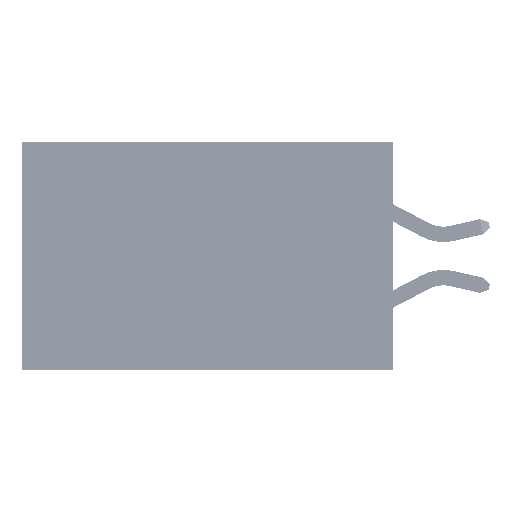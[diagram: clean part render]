
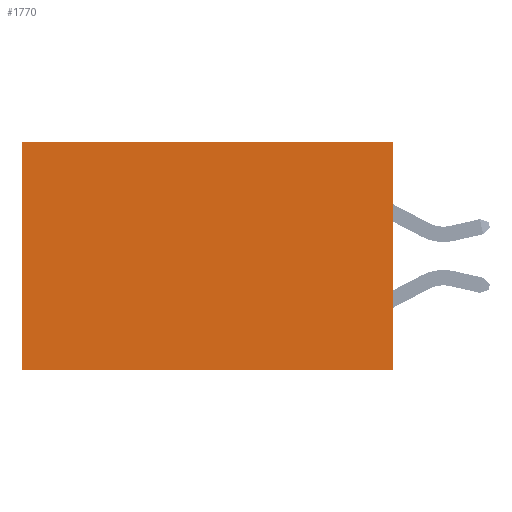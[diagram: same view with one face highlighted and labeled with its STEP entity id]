
A CAD part, left-side view. The second image highlights one B-rep face of the part: STEP entity #1770.
In plain terms, the highlighted planar face has unit normal (-1, 0, 0).
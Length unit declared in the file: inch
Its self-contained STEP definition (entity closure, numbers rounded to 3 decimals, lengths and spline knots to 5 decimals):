
#869 = VECTOR ( 'NONE', #29882, 39.37008 ) ;
#1770 = ADVANCED_FACE ( 'NONE', ( #36019 ), #12127, .F. ) ;
#2548 = EDGE_CURVE ( 'NONE', #43400, #11097, #41888, .T. ) ;
#6231 = CARTESIAN_POINT ( 'NONE',  ( 0.2875, 0.6, 0. ) ) ;
#7928 = EDGE_CURVE ( 'NONE', #30086, #43400, #29965, .T. ) ;
#8043 = EDGE_CURVE ( 'NONE', #30086, #38669, #17926, .T. ) ;
#9518 = VECTOR ( 'NONE', #36520, 39.37008 ) ;
#11097 = VERTEX_POINT ( 'NONE', #26124 ) ;
#11501 = EDGE_LOOP ( 'NONE', ( #35897, #20294, #34209, #25399 ) ) ;
#12127 = PLANE ( 'NONE',  #30588 ) ;
#17926 = LINE ( 'NONE', #28607, #9518 ) ;
#19720 = DIRECTION ( 'NONE',  ( 1., 0., 0. ) ) ;
#20294 = ORIENTED_EDGE ( 'NONE', *, *, #21108, .F. ) ;
#21108 = EDGE_CURVE ( 'NONE', #38669, #11097, #23764, .T. ) ;
#23764 = LINE ( 'NONE', #44851, #869 ) ;
#24514 = CARTESIAN_POINT ( 'NONE',  ( 0.2875, 0., -0.37 ) ) ;
#25399 = ORIENTED_EDGE ( 'NONE', *, *, #7928, .T. ) ;
#26124 = CARTESIAN_POINT ( 'NONE',  ( 0.2875, 0.6, -0.37 ) ) ;
#26771 = DIRECTION ( 'NONE',  ( 0., 0., -1. ) ) ;
#27889 = CARTESIAN_POINT ( 'NONE',  ( 0.2875, 0., 0. ) ) ;
#28607 = CARTESIAN_POINT ( 'NONE',  ( 0.2875, 0., 0. ) ) ;
#29882 = DIRECTION ( 'NONE',  ( 0., 1., 0. ) ) ;
#29965 = LINE ( 'NONE', #46790, #38418 ) ;
#30086 = VERTEX_POINT ( 'NONE', #27889 ) ;
#30588 = AXIS2_PLACEMENT_3D ( 'NONE', #46478, #19720, #26771 ) ;
#31828 = DIRECTION ( 'NONE',  ( 0., 1., 0. ) ) ;
#34209 = ORIENTED_EDGE ( 'NONE', *, *, #8043, .F. ) ;
#35166 = CARTESIAN_POINT ( 'NONE',  ( 0.2875, 0.6, 0. ) ) ;
#35897 = ORIENTED_EDGE ( 'NONE', *, *, #2548, .T. ) ;
#36019 = FACE_OUTER_BOUND ( 'NONE', #11501, .T. ) ;
#36520 = DIRECTION ( 'NONE',  ( 0., 0., -1. ) ) ;
#36664 = DIRECTION ( 'NONE',  ( 0., 0., -1. ) ) ;
#38418 = VECTOR ( 'NONE', #31828, 39.37008 ) ;
#38669 = VERTEX_POINT ( 'NONE', #24514 ) ;
#41888 = LINE ( 'NONE', #6231, #45546 ) ;
#43400 = VERTEX_POINT ( 'NONE', #35166 ) ;
#44851 = CARTESIAN_POINT ( 'NONE',  ( 0.2875, 0., -0.37 ) ) ;
#45546 = VECTOR ( 'NONE', #36664, 39.37008 ) ;
#46478 = CARTESIAN_POINT ( 'NONE',  ( 0.2875, 0., 0. ) ) ;
#46790 = CARTESIAN_POINT ( 'NONE',  ( 0.2875, 0., 0. ) ) ;
